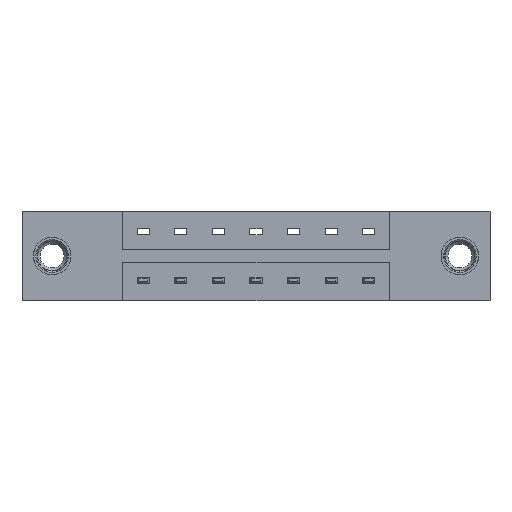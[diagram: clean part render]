
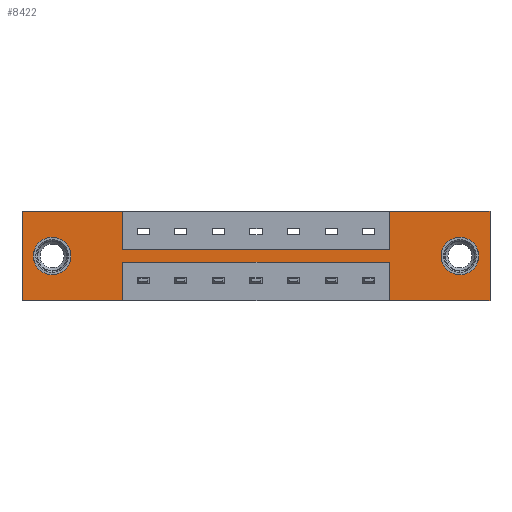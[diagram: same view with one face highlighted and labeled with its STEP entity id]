
A CAD part, front view. The second image highlights one B-rep face of the part: STEP entity #8422.
In plain terms, the highlighted planar face has unit normal (0, -1, 0).
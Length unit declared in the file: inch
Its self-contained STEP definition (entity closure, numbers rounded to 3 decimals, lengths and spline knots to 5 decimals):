
#8 = CARTESIAN_POINT ( 'NONE',  ( 0., 0., 0. ) ) ;
#81 = DIRECTION ( 'NONE',  ( 0., 0., -1. ) ) ;
#116 = DIRECTION ( 'NONE',  ( 0., 0., 1. ) ) ;
#127 = CIRCLE ( 'NONE', #4424, 0.078 ) ;
#133 = VECTOR ( 'NONE', #708, 39.37008 ) ;
#171 = LINE ( 'NONE', #4602, #1396 ) ;
#177 = CARTESIAN_POINT ( 'NONE',  ( 1.5225, 0., 0. ) ) ;
#208 = DIRECTION ( 'NONE',  ( 1., 0., 0. ) ) ;
#246 = DIRECTION ( 'NONE',  ( 0., 1., 0. ) ) ;
#348 = EDGE_CURVE ( 'NONE', #2812, #698, #3932, .T. ) ;
#498 = VERTEX_POINT ( 'NONE', #7848 ) ;
#600 = VECTOR ( 'NONE', #8893, 39.37008 ) ;
#604 = EDGE_CURVE ( 'NONE', #7344, #498, #2089, .T. ) ;
#695 = VECTOR ( 'NONE', #3413, 39.37008 ) ;
#698 = VERTEX_POINT ( 'NONE', #1942 ) ;
#708 = DIRECTION ( 'NONE',  ( -1., 0., 0. ) ) ;
#859 = LINE ( 'NONE', #8511, #7801 ) ;
#924 = ORIENTED_EDGE ( 'NONE', *, *, #4903, .F. ) ;
#986 = DIRECTION ( 'NONE',  ( 0., 1., 0. ) ) ;
#1012 = CARTESIAN_POINT ( 'NONE',  ( 1.5225, 0., -0.1585 ) ) ;
#1396 = VECTOR ( 'NONE', #7629, 39.37008 ) ;
#1414 = AXIS2_PLACEMENT_3D ( 'NONE', #3973, #986, #3531 ) ;
#1547 = VECTOR ( 'NONE', #116, 39.37008 ) ;
#1563 = CARTESIAN_POINT ( 'NONE',  ( 1.5225, 0., -0.2115 ) ) ;
#1598 = ORIENTED_EDGE ( 'NONE', *, *, #6407, .T. ) ;
#1626 = VECTOR ( 'NONE', #3623, 39.37008 ) ;
#1689 = CARTESIAN_POINT ( 'NONE',  ( 0.4175, 0., 0. ) ) ;
#1841 = CARTESIAN_POINT ( 'NONE',  ( 0.125, 0., -0.185 ) ) ;
#1942 = CARTESIAN_POINT ( 'NONE',  ( 1.94, 0., 0. ) ) ;
#1974 = EDGE_CURVE ( 'NONE', #9077, #5050, #859, .T. ) ;
#1984 = DIRECTION ( 'NONE',  ( 0., 0., 1. ) ) ;
#2089 = LINE ( 'NONE', #2678, #7619 ) ;
#2128 = VERTEX_POINT ( 'NONE', #8816 ) ;
#2217 = VECTOR ( 'NONE', #3737, 39.37008 ) ;
#2218 = ORIENTED_EDGE ( 'NONE', *, *, #3939, .F. ) ;
#2224 = CARTESIAN_POINT ( 'NONE',  ( 0., 0., -0.37 ) ) ;
#2243 = ORIENTED_EDGE ( 'NONE', *, *, #3744, .T. ) ;
#2458 = EDGE_CURVE ( 'NONE', #8919, #5212, #5600, .T. ) ;
#2468 = ORIENTED_EDGE ( 'NONE', *, *, #1974, .F. ) ;
#2503 = VERTEX_POINT ( 'NONE', #8841 ) ;
#2558 = ORIENTED_EDGE ( 'NONE', *, *, #8955, .F. ) ;
#2601 = VERTEX_POINT ( 'NONE', #3112 ) ;
#2620 = LINE ( 'NONE', #6617, #600 ) ;
#2678 = CARTESIAN_POINT ( 'NONE',  ( 0., 0., -0.37 ) ) ;
#2812 = VERTEX_POINT ( 'NONE', #177 ) ;
#2884 = CARTESIAN_POINT ( 'NONE',  ( 0.125, 0., -0.107 ) ) ;
#3096 = ORIENTED_EDGE ( 'NONE', *, *, #9504, .F. ) ;
#3112 = CARTESIAN_POINT ( 'NONE',  ( 0.4175, 0., -0.2115 ) ) ;
#3136 = DIRECTION ( 'NONE',  ( 0., 0., 1. ) ) ;
#3311 = ORIENTED_EDGE ( 'NONE', *, *, #4218, .F. ) ;
#3413 = DIRECTION ( 'NONE',  ( 0., 0., 1. ) ) ;
#3531 = DIRECTION ( 'NONE',  ( 0., 0., -1. ) ) ;
#3623 = DIRECTION ( 'NONE',  ( -1., 0., 0. ) ) ;
#3737 = DIRECTION ( 'NONE',  ( 1., 0., 0. ) ) ;
#3744 = EDGE_CURVE ( 'NONE', #3862, #2503, #127, .T. ) ;
#3855 = CARTESIAN_POINT ( 'NONE',  ( 0.125, 0., -0.263 ) ) ;
#3862 = VERTEX_POINT ( 'NONE', #6369 ) ;
#3932 = LINE ( 'NONE', #7706, #2217 ) ;
#3939 = EDGE_CURVE ( 'NONE', #7439, #2601, #7509, .T. ) ;
#3973 = CARTESIAN_POINT ( 'NONE',  ( 1.815, 0., -0.185 ) ) ;
#4218 = EDGE_CURVE ( 'NONE', #5050, #2128, #6496, .T. ) ;
#4228 = EDGE_CURVE ( 'NONE', #7609, #2812, #8440, .T. ) ;
#4424 = AXIS2_PLACEMENT_3D ( 'NONE', #8707, #5041, #9433 ) ;
#4602 = CARTESIAN_POINT ( 'NONE',  ( 0.4175, 0., -0.1585 ) ) ;
#4778 = CARTESIAN_POINT ( 'NONE',  ( 1.94, 0., -0.37 ) ) ;
#4903 = EDGE_CURVE ( 'NONE', #498, #9077, #6822, .T. ) ;
#4904 = CARTESIAN_POINT ( 'NONE',  ( 0., 0., 0. ) ) ;
#5024 = AXIS2_PLACEMENT_3D ( 'NONE', #1841, #246, #8607 ) ;
#5041 = DIRECTION ( 'NONE',  ( 0., 1., 0. ) ) ;
#5050 = VERTEX_POINT ( 'NONE', #1689 ) ;
#5078 = CARTESIAN_POINT ( 'NONE',  ( 0.125, 0., -0.185 ) ) ;
#5127 = DIRECTION ( 'NONE',  ( -1., 0., 0. ) ) ;
#5199 = CARTESIAN_POINT ( 'NONE',  ( 1.5225, 0., -0.2115 ) ) ;
#5206 = EDGE_LOOP ( 'NONE', ( #1598, #7890 ) ) ;
#5212 = VERTEX_POINT ( 'NONE', #2884 ) ;
#5575 = EDGE_CURVE ( 'NONE', #2503, #3862, #9010, .T. ) ;
#5594 = CARTESIAN_POINT ( 'NONE',  ( 0.4175, 0., -0.1585 ) ) ;
#5600 = CIRCLE ( 'NONE', #8147, 0.078 ) ;
#5630 = EDGE_LOOP ( 'NONE', ( #2243, #6907 ) ) ;
#5753 = EDGE_CURVE ( 'NONE', #9401, #9254, #7446, .T. ) ;
#5779 = ORIENTED_EDGE ( 'NONE', *, *, #4228, .F. ) ;
#5838 = CARTESIAN_POINT ( 'NONE',  ( 1.5225, 0., -0.37 ) ) ;
#5880 = CARTESIAN_POINT ( 'NONE',  ( 0.4175, 0., -0.2115 ) ) ;
#5886 = EDGE_LOOP ( 'NONE', ( #2558, #7323, #3096, #8650, #5779, #9265, #3311, #2468, #924, #6861, #6185, #2218 ) ) ;
#6013 = DIRECTION ( 'NONE',  ( 0., 0., -1. ) ) ;
#6185 = ORIENTED_EDGE ( 'NONE', *, *, #6688, .F. ) ;
#6221 = VECTOR ( 'NONE', #3136, 39.37008 ) ;
#6369 = CARTESIAN_POINT ( 'NONE',  ( 1.815, 0., -0.107 ) ) ;
#6407 = EDGE_CURVE ( 'NONE', #5212, #8919, #7703, .T. ) ;
#6496 = LINE ( 'NONE', #5594, #7979 ) ;
#6617 = CARTESIAN_POINT ( 'NONE',  ( 1.94, 0., 0. ) ) ;
#6688 = EDGE_CURVE ( 'NONE', #2601, #7344, #7052, .T. ) ;
#6717 = FACE_BOUND ( 'NONE', #5206, .T. ) ;
#6763 = DIRECTION ( 'NONE',  ( 0., -1., 0. ) ) ;
#6822 = LINE ( 'NONE', #8, #6221 ) ;
#6861 = ORIENTED_EDGE ( 'NONE', *, *, #604, .F. ) ;
#6881 = LINE ( 'NONE', #1563, #1547 ) ;
#6907 = ORIENTED_EDGE ( 'NONE', *, *, #5575, .T. ) ;
#7052 = LINE ( 'NONE', #8640, #9281 ) ;
#7323 = ORIENTED_EDGE ( 'NONE', *, *, #5753, .F. ) ;
#7344 = VERTEX_POINT ( 'NONE', #7432 ) ;
#7432 = CARTESIAN_POINT ( 'NONE',  ( 0.4175, 0., -0.37 ) ) ;
#7439 = VERTEX_POINT ( 'NONE', #5199 ) ;
#7446 = LINE ( 'NONE', #2224, #1626 ) ;
#7501 = PLANE ( 'NONE',  #8523 ) ;
#7509 = LINE ( 'NONE', #5880, #133 ) ;
#7609 = VERTEX_POINT ( 'NONE', #1012 ) ;
#7619 = VECTOR ( 'NONE', #5127, 39.37008 ) ;
#7629 = DIRECTION ( 'NONE',  ( 1., 0., 0. ) ) ;
#7703 = CIRCLE ( 'NONE', #5024, 0.078 ) ;
#7706 = CARTESIAN_POINT ( 'NONE',  ( 0., 0., 0. ) ) ;
#7801 = VECTOR ( 'NONE', #208, 39.37008 ) ;
#7848 = CARTESIAN_POINT ( 'NONE',  ( 0., 0., -0.37 ) ) ;
#7890 = ORIENTED_EDGE ( 'NONE', *, *, #2458, .T. ) ;
#7979 = VECTOR ( 'NONE', #81, 39.37008 ) ;
#8043 = DIRECTION ( 'NONE',  ( 0., 1., 0. ) ) ;
#8147 = AXIS2_PLACEMENT_3D ( 'NONE', #5078, #8043, #1984 ) ;
#8396 = CARTESIAN_POINT ( 'NONE',  ( 1.5225, 0., -0.1585 ) ) ;
#8422 = ADVANCED_FACE ( 'NONE', ( #8939, #6717, #9732 ), #7501, .T. ) ;
#8440 = LINE ( 'NONE', #8396, #695 ) ;
#8511 = CARTESIAN_POINT ( 'NONE',  ( 0., 0., 0. ) ) ;
#8523 = AXIS2_PLACEMENT_3D ( 'NONE', #9780, #6763, #6013 ) ;
#8592 = DIRECTION ( 'NONE',  ( 0., 0., -1. ) ) ;
#8607 = DIRECTION ( 'NONE',  ( 0., 0., 1. ) ) ;
#8640 = CARTESIAN_POINT ( 'NONE',  ( 0.4175, 0., -0.2115 ) ) ;
#8650 = ORIENTED_EDGE ( 'NONE', *, *, #348, .F. ) ;
#8707 = CARTESIAN_POINT ( 'NONE',  ( 1.815, 0., -0.185 ) ) ;
#8816 = CARTESIAN_POINT ( 'NONE',  ( 0.4175, 0., -0.1585 ) ) ;
#8841 = CARTESIAN_POINT ( 'NONE',  ( 1.815, 0., -0.263 ) ) ;
#8893 = DIRECTION ( 'NONE',  ( 0., 0., -1. ) ) ;
#8919 = VERTEX_POINT ( 'NONE', #3855 ) ;
#8939 = FACE_BOUND ( 'NONE', #5630, .T. ) ;
#8955 = EDGE_CURVE ( 'NONE', #9254, #7439, #6881, .T. ) ;
#8959 = EDGE_CURVE ( 'NONE', #2128, #7609, #171, .T. ) ;
#9010 = CIRCLE ( 'NONE', #1414, 0.078 ) ;
#9077 = VERTEX_POINT ( 'NONE', #4904 ) ;
#9254 = VERTEX_POINT ( 'NONE', #5838 ) ;
#9265 = ORIENTED_EDGE ( 'NONE', *, *, #8959, .F. ) ;
#9281 = VECTOR ( 'NONE', #8592, 39.37008 ) ;
#9401 = VERTEX_POINT ( 'NONE', #4778 ) ;
#9433 = DIRECTION ( 'NONE',  ( 0., 0., -1. ) ) ;
#9504 = EDGE_CURVE ( 'NONE', #698, #9401, #2620, .T. ) ;
#9732 = FACE_OUTER_BOUND ( 'NONE', #5886, .T. ) ;
#9780 = CARTESIAN_POINT ( 'NONE',  ( 0., 0., -0.37 ) ) ;
